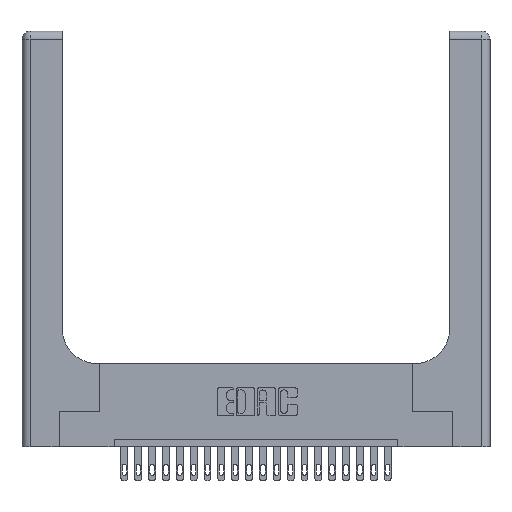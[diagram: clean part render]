
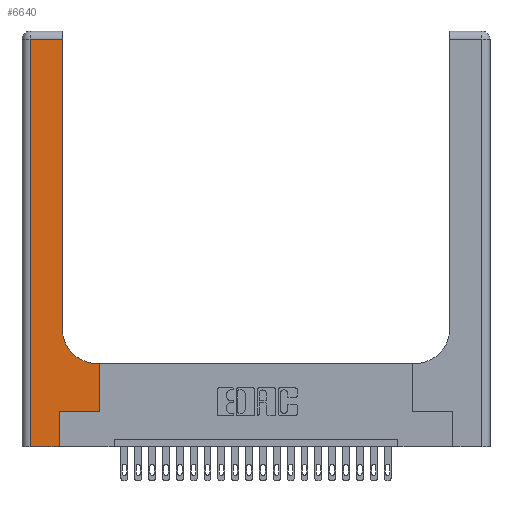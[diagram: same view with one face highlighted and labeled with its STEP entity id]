
A CAD part, top view. The second image highlights one B-rep face of the part: STEP entity #6640.
In plain terms, the highlighted planar face has unit normal (0, 0, 1).
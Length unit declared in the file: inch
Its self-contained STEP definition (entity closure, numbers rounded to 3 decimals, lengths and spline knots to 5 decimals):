
#43 = CARTESIAN_POINT ( 'NONE',  ( 0.5585, 0.6, 0.37 ) ) ;
#485 = DIRECTION ( 'NONE',  ( 0., 1., 0. ) ) ;
#585 = VERTEX_POINT ( 'NONE', #6174 ) ;
#828 = CARTESIAN_POINT ( 'NONE',  ( 0.269, 0.25, 0.37 ) ) ;
#918 = EDGE_CURVE ( 'NONE', #6673, #11008, #4599, .T. ) ;
#1436 = AXIS2_PLACEMENT_3D ( 'NONE', #2702, #15154, #11814 ) ;
#1645 = VERTEX_POINT ( 'NONE', #43 ) ;
#2296 = VECTOR ( 'NONE', #11731, 39.37008 ) ;
#2702 = CARTESIAN_POINT ( 'NONE',  ( 0.5415, 0.85, 0.37 ) ) ;
#2834 = EDGE_LOOP ( 'NONE', ( #18725, #14135, #12095, #22472, #7129, #13888, #21305, #9527, #5603 ) ) ;
#2868 = DIRECTION ( 'NONE',  ( 1., 0., 0. ) ) ;
#2910 = DIRECTION ( 'NONE',  ( 0., -1., 0. ) ) ;
#3188 = LINE ( 'NONE', #19291, #9613 ) ;
#3335 = VECTOR ( 'NONE', #485, 39.37008 ) ;
#3409 = VERTEX_POINT ( 'NONE', #21285 ) ;
#3822 = CARTESIAN_POINT ( 'NONE',  ( 0.269, 0., 0.37 ) ) ;
#4060 = CARTESIAN_POINT ( 'NONE',  ( 0.06, 0., 0.37 ) ) ;
#4513 = EDGE_CURVE ( 'NONE', #1645, #16819, #3188, .T. ) ;
#4599 = LINE ( 'NONE', #9492, #11844 ) ;
#4864 = LINE ( 'NONE', #16978, #16269 ) ;
#5326 = AXIS2_PLACEMENT_3D ( 'NONE', #16049, #19801, #7279 ) ;
#5521 = DIRECTION ( 'NONE',  ( 0., 1., 0. ) ) ;
#5603 = ORIENTED_EDGE ( 'NONE', *, *, #16126, .T. ) ;
#6174 = CARTESIAN_POINT ( 'NONE',  ( 0.2915, 0.85, 0.37 ) ) ;
#6636 = LINE ( 'NONE', #7432, #20004 ) ;
#6640 = ADVANCED_FACE ( 'NONE', ( #21522 ), #17924, .F. ) ;
#6673 = VERTEX_POINT ( 'NONE', #3822 ) ;
#7129 = ORIENTED_EDGE ( 'NONE', *, *, #918, .T. ) ;
#7245 = VERTEX_POINT ( 'NONE', #12392 ) ;
#7279 = DIRECTION ( 'NONE',  ( -1., 0., 0. ) ) ;
#7365 = DIRECTION ( 'NONE',  ( -1., 0., 0. ) ) ;
#7432 = CARTESIAN_POINT ( 'NONE',  ( 0., 2.94, 0.37 ) ) ;
#7529 = CARTESIAN_POINT ( 'NONE',  ( 0.2915, 3., 0.37 ) ) ;
#9279 = LINE ( 'NONE', #13369, #13444 ) ;
#9492 = CARTESIAN_POINT ( 'NONE',  ( 0.269, 0., 0.37 ) ) ;
#9527 = ORIENTED_EDGE ( 'NONE', *, *, #4513, .T. ) ;
#9613 = VECTOR ( 'NONE', #10871, 39.37008 ) ;
#10795 = VERTEX_POINT ( 'NONE', #21260 ) ;
#10871 = DIRECTION ( 'NONE',  ( -1., 0., 0. ) ) ;
#11008 = VERTEX_POINT ( 'NONE', #828 ) ;
#11731 = DIRECTION ( 'NONE',  ( 0., 1., 0. ) ) ;
#11814 = DIRECTION ( 'NONE',  ( 1., 0., 0. ) ) ;
#11844 = VECTOR ( 'NONE', #5521, 39.37008 ) ;
#11987 = EDGE_CURVE ( 'NONE', #17386, #6673, #9279, .T. ) ;
#12095 = ORIENTED_EDGE ( 'NONE', *, *, #19237, .T. ) ;
#12392 = CARTESIAN_POINT ( 'NONE',  ( 0.2915, 2.94, 0.37 ) ) ;
#12741 = LINE ( 'NONE', #16371, #16095 ) ;
#12870 = DIRECTION ( 'NONE',  ( 1., 0., 0. ) ) ;
#13369 = CARTESIAN_POINT ( 'NONE',  ( 0., 0., 0.37 ) ) ;
#13444 = VECTOR ( 'NONE', #2868, 39.37008 ) ;
#13633 = CARTESIAN_POINT ( 'NONE',  ( 0.5415, 0.6, 0.37 ) ) ;
#13888 = ORIENTED_EDGE ( 'NONE', *, *, #14674, .T. ) ;
#14135 = ORIENTED_EDGE ( 'NONE', *, *, #17313, .T. ) ;
#14192 = EDGE_CURVE ( 'NONE', #585, #7245, #15295, .T. ) ;
#14674 = EDGE_CURVE ( 'NONE', #11008, #3409, #12741, .T. ) ;
#15154 = DIRECTION ( 'NONE',  ( 0., 0., -1. ) ) ;
#15295 = LINE ( 'NONE', #7529, #3335 ) ;
#16049 = CARTESIAN_POINT ( 'NONE',  ( 0., 3., 0.37 ) ) ;
#16095 = VECTOR ( 'NONE', #12870, 39.37008 ) ;
#16126 = EDGE_CURVE ( 'NONE', #16819, #585, #16702, .T. ) ;
#16269 = VECTOR ( 'NONE', #2910, 39.37008 ) ;
#16371 = CARTESIAN_POINT ( 'NONE',  ( 0.269, 0.25, 0.37 ) ) ;
#16702 = CIRCLE ( 'NONE', #1436, 0.25 ) ;
#16819 = VERTEX_POINT ( 'NONE', #13633 ) ;
#16978 = CARTESIAN_POINT ( 'NONE',  ( 0.06, 3., 0.37 ) ) ;
#17313 = EDGE_CURVE ( 'NONE', #7245, #10795, #6636, .T. ) ;
#17386 = VERTEX_POINT ( 'NONE', #4060 ) ;
#17638 = LINE ( 'NONE', #18892, #2296 ) ;
#17924 = PLANE ( 'NONE',  #5326 ) ;
#18725 = ORIENTED_EDGE ( 'NONE', *, *, #14192, .T. ) ;
#18892 = CARTESIAN_POINT ( 'NONE',  ( 0.5585, 0.25, 0.37 ) ) ;
#19237 = EDGE_CURVE ( 'NONE', #10795, #17386, #4864, .T. ) ;
#19291 = CARTESIAN_POINT ( 'NONE',  ( 0.2915, 0.6, 0.37 ) ) ;
#19801 = DIRECTION ( 'NONE',  ( 0., 0., -1. ) ) ;
#20004 = VECTOR ( 'NONE', #7365, 39.37008 ) ;
#21260 = CARTESIAN_POINT ( 'NONE',  ( 0.06, 2.94, 0.37 ) ) ;
#21285 = CARTESIAN_POINT ( 'NONE',  ( 0.5585, 0.25, 0.37 ) ) ;
#21305 = ORIENTED_EDGE ( 'NONE', *, *, #22743, .T. ) ;
#21522 = FACE_OUTER_BOUND ( 'NONE', #2834, .T. ) ;
#22472 = ORIENTED_EDGE ( 'NONE', *, *, #11987, .T. ) ;
#22743 = EDGE_CURVE ( 'NONE', #3409, #1645, #17638, .T. ) ;
